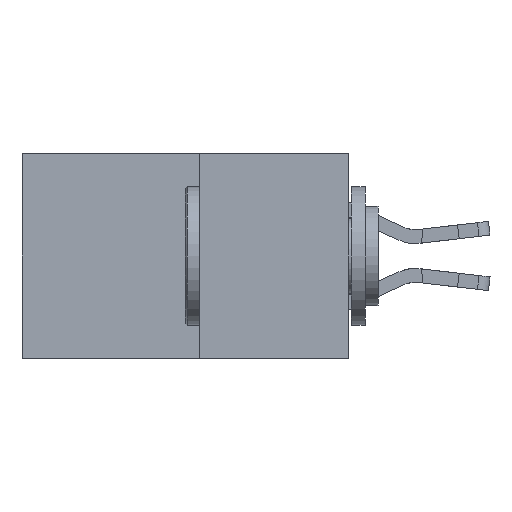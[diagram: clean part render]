
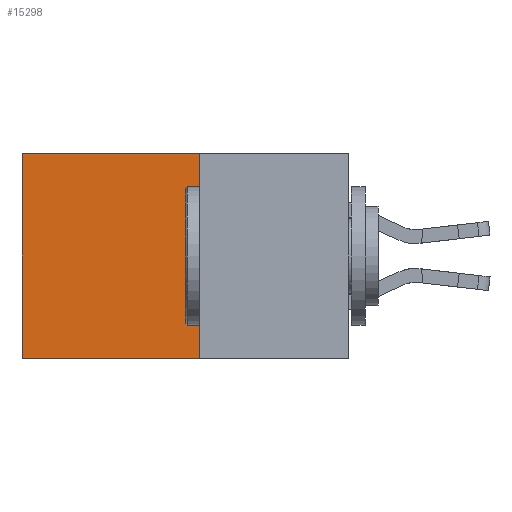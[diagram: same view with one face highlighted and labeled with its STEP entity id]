
A CAD part, left-side view. The second image highlights one B-rep face of the part: STEP entity #15298.
In plain terms, the highlighted planar face has unit normal (-1, 0, 0).
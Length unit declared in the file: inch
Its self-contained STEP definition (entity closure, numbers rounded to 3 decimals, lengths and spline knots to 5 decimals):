
#73 = CARTESIAN_POINT ( 'NONE',  ( 0.277, 0.27, -0.37 ) ) ;
#402 = VECTOR ( 'NONE', #515, 39.37008 ) ;
#413 = CARTESIAN_POINT ( 'NONE',  ( 0.277, 0.27, -0.37 ) ) ;
#515 = DIRECTION ( 'NONE',  ( 0., 1., 0. ) ) ;
#554 = VECTOR ( 'NONE', #1444, 39.37008 ) ;
#604 = DIRECTION ( 'NONE',  ( 1., 0., 0. ) ) ;
#1444 = DIRECTION ( 'NONE',  ( 0., 0., -1. ) ) ;
#1516 = LINE ( 'NONE', #14119, #13843 ) ;
#1745 = DIRECTION ( 'NONE',  ( 0., 0., -1. ) ) ;
#2454 = CARTESIAN_POINT ( 'NONE',  ( 0.277, 0.59, 0. ) ) ;
#2853 = CARTESIAN_POINT ( 'NONE',  ( 0.277, 0.59, -0.37 ) ) ;
#3820 = PLANE ( 'NONE',  #19999 ) ;
#4329 = EDGE_CURVE ( 'NONE', #18527, #10059, #1516, .T. ) ;
#4868 = CARTESIAN_POINT ( 'NONE',  ( 0.277, 0.27, 0. ) ) ;
#5427 = LINE ( 'NONE', #73, #17717 ) ;
#5759 = ORIENTED_EDGE ( 'NONE', *, *, #13249, .F. ) ;
#9434 = EDGE_CURVE ( 'NONE', #18071, #10059, #13405, .T. ) ;
#10059 = VERTEX_POINT ( 'NONE', #2853 ) ;
#10323 = CARTESIAN_POINT ( 'NONE',  ( 0.277, 0.27, -0.37 ) ) ;
#11017 = EDGE_CURVE ( 'NONE', #13221, #18071, #13257, .T. ) ;
#11809 = CARTESIAN_POINT ( 'NONE',  ( 0.277, 0.27, 0. ) ) ;
#11894 = DIRECTION ( 'NONE',  ( 0., 0., -1. ) ) ;
#13019 = ORIENTED_EDGE ( 'NONE', *, *, #11017, .T. ) ;
#13221 = VERTEX_POINT ( 'NONE', #4868 ) ;
#13249 = EDGE_CURVE ( 'NONE', #13221, #18527, #5427, .T. ) ;
#13257 = LINE ( 'NONE', #11809, #402 ) ;
#13405 = LINE ( 'NONE', #20552, #554 ) ;
#13843 = VECTOR ( 'NONE', #13998, 39.37008 ) ;
#13998 = DIRECTION ( 'NONE',  ( 0., 1., 0. ) ) ;
#14116 = FACE_OUTER_BOUND ( 'NONE', #17560, .T. ) ;
#14119 = CARTESIAN_POINT ( 'NONE',  ( 0.277, 0.27, -0.37 ) ) ;
#15298 = ADVANCED_FACE ( 'NONE', ( #14116 ), #3820, .F. ) ;
#15846 = ORIENTED_EDGE ( 'NONE', *, *, #4329, .F. ) ;
#17560 = EDGE_LOOP ( 'NONE', ( #18114, #15846, #5759, #13019 ) ) ;
#17717 = VECTOR ( 'NONE', #1745, 39.37008 ) ;
#18071 = VERTEX_POINT ( 'NONE', #2454 ) ;
#18114 = ORIENTED_EDGE ( 'NONE', *, *, #9434, .T. ) ;
#18527 = VERTEX_POINT ( 'NONE', #413 ) ;
#19999 = AXIS2_PLACEMENT_3D ( 'NONE', #10323, #604, #11894 ) ;
#20552 = CARTESIAN_POINT ( 'NONE',  ( 0.277, 0.59, -0.37 ) ) ;
